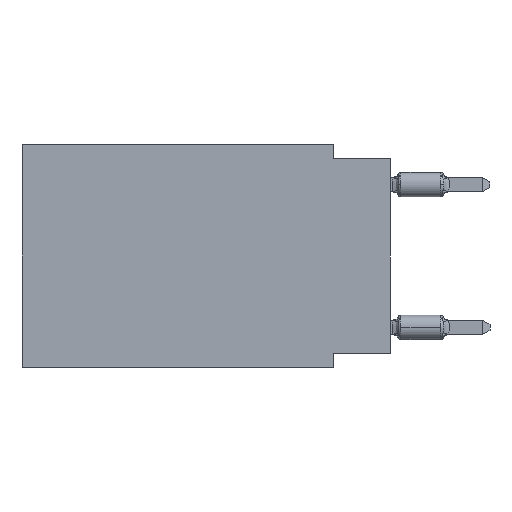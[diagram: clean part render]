
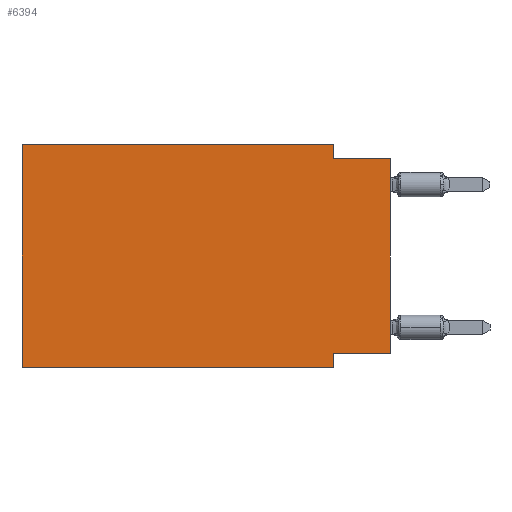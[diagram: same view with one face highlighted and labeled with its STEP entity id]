
A CAD part, left-side view. The second image highlights one B-rep face of the part: STEP entity #6394.
In plain terms, the highlighted planar face has unit normal (-1, 0, 0).
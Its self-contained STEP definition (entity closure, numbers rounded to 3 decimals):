
#330 = DIRECTION ( 'NONE',  ( 0., 0., -1. ) ) ;
#433 = CARTESIAN_POINT ( 'NONE',  ( 0., 2.54, -9.906 ) ) ;
#693 = CARTESIAN_POINT ( 'NONE',  ( 0., 16.383, 0. ) ) ;
#1211 = EDGE_CURVE ( 'NONE', #15030, #14905, #7630, .T. ) ;
#1316 = VECTOR ( 'NONE', #4318, 1000. ) ;
#1456 = LINE ( 'NONE', #433, #12150 ) ;
#1538 = DIRECTION ( 'NONE',  ( 0., 0., -1. ) ) ;
#1814 = ORIENTED_EDGE ( 'NONE', *, *, #10074, .F. ) ;
#2804 = ORIENTED_EDGE ( 'NONE', *, *, #6307, .T. ) ;
#3194 = CARTESIAN_POINT ( 'NONE',  ( 0., 2.54, 0. ) ) ;
#3203 = VECTOR ( 'NONE', #11532, 1000. ) ;
#3219 = VECTOR ( 'NONE', #8942, 1000. ) ;
#3345 = DIRECTION ( 'NONE',  ( 0., 0., -1. ) ) ;
#4318 = DIRECTION ( 'NONE',  ( 0., 0., 1. ) ) ;
#4428 = CARTESIAN_POINT ( 'NONE',  ( 0., 2.54, -9.271 ) ) ;
#5127 = ORIENTED_EDGE ( 'NONE', *, *, #10890, .F. ) ;
#5149 = VERTEX_POINT ( 'NONE', #3194 ) ;
#5255 = ORIENTED_EDGE ( 'NONE', *, *, #1211, .T. ) ;
#5506 = LINE ( 'NONE', #10377, #3219 ) ;
#5565 = VECTOR ( 'NONE', #6261, 1000. ) ;
#5660 = FACE_OUTER_BOUND ( 'NONE', #10575, .T. ) ;
#5740 = CARTESIAN_POINT ( 'NONE',  ( 0., 16.383, 0. ) ) ;
#5895 = LINE ( 'NONE', #10764, #11574 ) ;
#6128 = CARTESIAN_POINT ( 'NONE',  ( 0., 0., -0.635 ) ) ;
#6261 = DIRECTION ( 'NONE',  ( 0., -1., 0. ) ) ;
#6307 = EDGE_CURVE ( 'NONE', #8545, #13473, #8142, .T. ) ;
#6394 = ADVANCED_FACE ( 'NONE', ( #5660 ), #14351, .F. ) ;
#6480 = ORIENTED_EDGE ( 'NONE', *, *, #15501, .F. ) ;
#7180 = EDGE_CURVE ( 'NONE', #10827, #5149, #7956, .T. ) ;
#7286 = CARTESIAN_POINT ( 'NONE',  ( 0., 16.383, -9.906 ) ) ;
#7630 = LINE ( 'NONE', #13520, #5565 ) ;
#7741 = EDGE_CURVE ( 'NONE', #8545, #11308, #5506, .T. ) ;
#7956 = LINE ( 'NONE', #693, #3203 ) ;
#8142 = LINE ( 'NONE', #9258, #1316 ) ;
#8501 = LINE ( 'NONE', #12003, #14347 ) ;
#8545 = VERTEX_POINT ( 'NONE', #8748 ) ;
#8619 = ORIENTED_EDGE ( 'NONE', *, *, #7180, .F. ) ;
#8748 = CARTESIAN_POINT ( 'NONE',  ( 0., 0., -9.271 ) ) ;
#8942 = DIRECTION ( 'NONE',  ( 0., 1., 0. ) ) ;
#9258 = CARTESIAN_POINT ( 'NONE',  ( 0., 0., 0. ) ) ;
#9410 = CARTESIAN_POINT ( 'NONE',  ( 0., 16.383, 0. ) ) ;
#9764 = DIRECTION ( 'NONE',  ( 0., -1., 0. ) ) ;
#9985 = CARTESIAN_POINT ( 'NONE',  ( 0., 2.54, -0.635 ) ) ;
#10074 = EDGE_CURVE ( 'NONE', #13022, #13473, #8501, .T. ) ;
#10377 = CARTESIAN_POINT ( 'NONE',  ( 0., 0., -9.271 ) ) ;
#10575 = EDGE_LOOP ( 'NONE', ( #2804, #1814, #6480, #8619, #5127, #5255, #13479, #11400 ) ) ;
#10764 = CARTESIAN_POINT ( 'NONE',  ( 0., 16.383, 0. ) ) ;
#10827 = VERTEX_POINT ( 'NONE', #9410 ) ;
#10890 = EDGE_CURVE ( 'NONE', #15030, #10827, #5895, .T. ) ;
#11308 = VERTEX_POINT ( 'NONE', #4428 ) ;
#11400 = ORIENTED_EDGE ( 'NONE', *, *, #7741, .F. ) ;
#11532 = DIRECTION ( 'NONE',  ( 0., -1., 0. ) ) ;
#11574 = VECTOR ( 'NONE', #15628, 1000. ) ;
#11862 = CARTESIAN_POINT ( 'NONE',  ( 0., 2.54, -9.906 ) ) ;
#12003 = CARTESIAN_POINT ( 'NONE',  ( 0., 0., -0.635 ) ) ;
#12150 = VECTOR ( 'NONE', #1538, 1000. ) ;
#12369 = LINE ( 'NONE', #14930, #12697 ) ;
#12697 = VECTOR ( 'NONE', #330, 1000. ) ;
#13022 = VERTEX_POINT ( 'NONE', #9985 ) ;
#13473 = VERTEX_POINT ( 'NONE', #6128 ) ;
#13479 = ORIENTED_EDGE ( 'NONE', *, *, #15175, .F. ) ;
#13520 = CARTESIAN_POINT ( 'NONE',  ( 0., 16.383, -9.906 ) ) ;
#14274 = DIRECTION ( 'NONE',  ( 1., 0., 0. ) ) ;
#14347 = VECTOR ( 'NONE', #9764, 1000. ) ;
#14351 = PLANE ( 'NONE',  #14392 ) ;
#14392 = AXIS2_PLACEMENT_3D ( 'NONE', #5740, #14274, #3345 ) ;
#14905 = VERTEX_POINT ( 'NONE', #11862 ) ;
#14930 = CARTESIAN_POINT ( 'NONE',  ( 0., 2.54, 0. ) ) ;
#15030 = VERTEX_POINT ( 'NONE', #7286 ) ;
#15175 = EDGE_CURVE ( 'NONE', #11308, #14905, #1456, .T. ) ;
#15501 = EDGE_CURVE ( 'NONE', #5149, #13022, #12369, .T. ) ;
#15628 = DIRECTION ( 'NONE',  ( 0., 0., 1. ) ) ;
